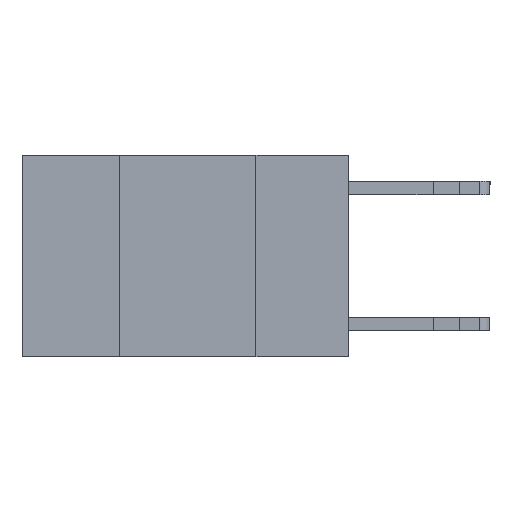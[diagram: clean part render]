
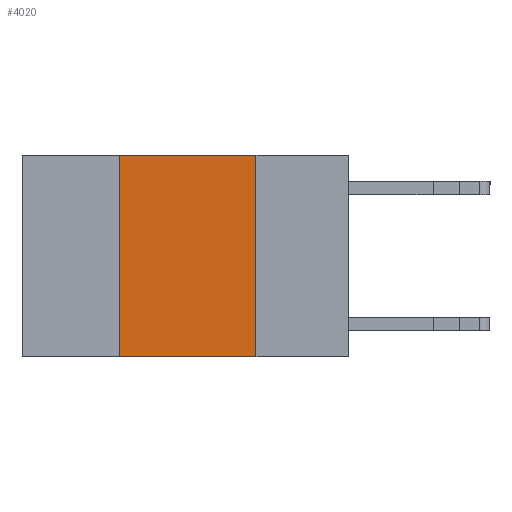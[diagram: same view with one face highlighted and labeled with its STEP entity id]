
A CAD part, left-side view. The second image highlights one B-rep face of the part: STEP entity #4020.
In plain terms, the highlighted planar face has unit normal (-1, 0, 0).
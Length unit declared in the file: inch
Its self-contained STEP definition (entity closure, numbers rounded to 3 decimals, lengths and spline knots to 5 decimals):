
#81 = CARTESIAN_POINT ( 'NONE',  ( 0., 0.6, 0. ) ) ;
#646 = ORIENTED_EDGE ( 'NONE', *, *, #1285, .F. ) ;
#1133 = PLANE ( 'NONE',  #3307 ) ;
#1156 = VECTOR ( 'NONE', #2698, 39.37008 ) ;
#1198 = DIRECTION ( 'NONE',  ( 0., -1., 0. ) ) ;
#1285 = EDGE_CURVE ( 'NONE', #1586, #3783, #7478, .T. ) ;
#1586 = VERTEX_POINT ( 'NONE', #10862 ) ;
#1956 = CARTESIAN_POINT ( 'NONE',  ( 0., 0.42, 0. ) ) ;
#1990 = FACE_OUTER_BOUND ( 'NONE', #10255, .T. ) ;
#2333 = ORIENTED_EDGE ( 'NONE', *, *, #10338, .F. ) ;
#2698 = DIRECTION ( 'NONE',  ( 0., -1., 0. ) ) ;
#3043 = EDGE_CURVE ( 'NONE', #10564, #1586, #6619, .T. ) ;
#3307 = AXIS2_PLACEMENT_3D ( 'NONE', #7540, #5665, #9350 ) ;
#3783 = VERTEX_POINT ( 'NONE', #9118 ) ;
#4020 = ADVANCED_FACE ( 'NONE', ( #1990 ), #1133, .F. ) ;
#4739 = DIRECTION ( 'NONE',  ( 0., 0., -1. ) ) ;
#4805 = LINE ( 'NONE', #11350, #11585 ) ;
#4984 = DIRECTION ( 'NONE',  ( 0., 0., 1. ) ) ;
#5369 = VECTOR ( 'NONE', #4739, 39.37008 ) ;
#5462 = EDGE_CURVE ( 'NONE', #11592, #3783, #5962, .T. ) ;
#5665 = DIRECTION ( 'NONE',  ( 1., 0., 0. ) ) ;
#5905 = CARTESIAN_POINT ( 'NONE',  ( 0., 0.42, -0.37 ) ) ;
#5962 = LINE ( 'NONE', #11478, #8522 ) ;
#6619 = LINE ( 'NONE', #81, #1156 ) ;
#7424 = CARTESIAN_POINT ( 'NONE',  ( 0., 0.17, 0. ) ) ;
#7478 = LINE ( 'NONE', #7424, #5369 ) ;
#7540 = CARTESIAN_POINT ( 'NONE',  ( 0., 0.6, 0. ) ) ;
#8373 = ORIENTED_EDGE ( 'NONE', *, *, #3043, .F. ) ;
#8422 = ORIENTED_EDGE ( 'NONE', *, *, #5462, .T. ) ;
#8522 = VECTOR ( 'NONE', #1198, 39.37008 ) ;
#9118 = CARTESIAN_POINT ( 'NONE',  ( 0., 0.17, -0.37 ) ) ;
#9350 = DIRECTION ( 'NONE',  ( 0., 0., -1. ) ) ;
#10255 = EDGE_LOOP ( 'NONE', ( #646, #8373, #2333, #8422 ) ) ;
#10338 = EDGE_CURVE ( 'NONE', #11592, #10564, #4805, .T. ) ;
#10564 = VERTEX_POINT ( 'NONE', #1956 ) ;
#10862 = CARTESIAN_POINT ( 'NONE',  ( 0., 0.17, 0. ) ) ;
#11350 = CARTESIAN_POINT ( 'NONE',  ( 0., 0.42, 0. ) ) ;
#11478 = CARTESIAN_POINT ( 'NONE',  ( 0., 0.6, -0.37 ) ) ;
#11585 = VECTOR ( 'NONE', #4984, 39.37008 ) ;
#11592 = VERTEX_POINT ( 'NONE', #5905 ) ;
